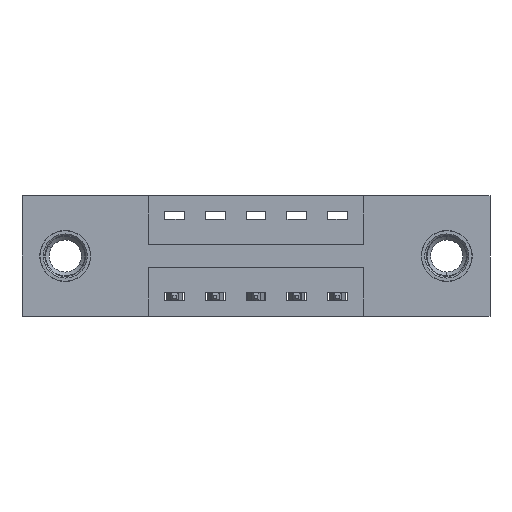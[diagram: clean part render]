
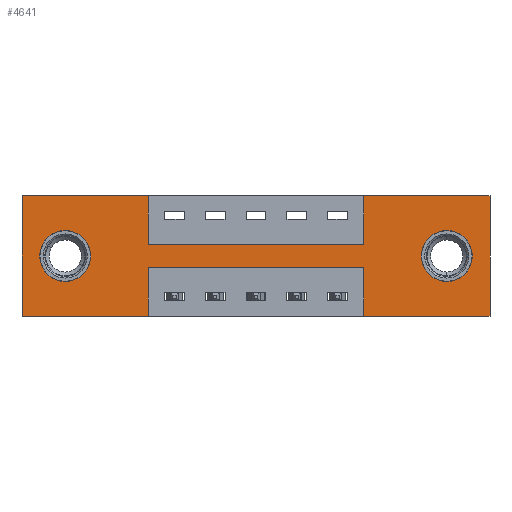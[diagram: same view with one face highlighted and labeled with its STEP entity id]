
A CAD part, front view. The second image highlights one B-rep face of the part: STEP entity #4641.
In plain terms, the highlighted planar face has unit normal (0, -1, 0).
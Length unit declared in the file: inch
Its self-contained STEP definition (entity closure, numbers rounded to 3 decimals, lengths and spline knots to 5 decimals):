
#1 = EDGE_CURVE ( 'NONE', #2073, #1929, #1153, .T. ) ;
#75 = VERTEX_POINT ( 'NONE', #7595 ) ;
#140 = DIRECTION ( 'NONE',  ( 0., 1., 0. ) ) ;
#154 = DIRECTION ( 'NONE',  ( 0., 0., 1. ) ) ;
#171 = CARTESIAN_POINT ( 'NONE',  ( 0.3875, 0., -0.15 ) ) ;
#267 = CARTESIAN_POINT ( 'NONE',  ( 1.3025, 0., -0.185 ) ) ;
#452 = EDGE_CURVE ( 'NONE', #1889, #619, #5421, .T. ) ;
#479 = FACE_OUTER_BOUND ( 'NONE', #673, .T. ) ;
#546 = EDGE_CURVE ( 'NONE', #6700, #4096, #1710, .T. ) ;
#568 = CARTESIAN_POINT ( 'NONE',  ( 0., 0., -0.37 ) ) ;
#619 = VERTEX_POINT ( 'NONE', #7642 ) ;
#673 = EDGE_LOOP ( 'NONE', ( #8582, #4911, #8316, #1388, #771, #6032, #5926, #6555, #3465, #4048, #6415, #8105 ) ) ;
#771 = ORIENTED_EDGE ( 'NONE', *, *, #8049, .F. ) ;
#792 = DIRECTION ( 'NONE',  ( 0., 0., -1. ) ) ;
#867 = CIRCLE ( 'NONE', #6271, 0.078 ) ;
#880 = DIRECTION ( 'NONE',  ( 0., 0., 1. ) ) ;
#926 = EDGE_CURVE ( 'NONE', #4603, #1766, #2413, .T. ) ;
#928 = CARTESIAN_POINT ( 'NONE',  ( 0.1325, 0., -0.185 ) ) ;
#943 = ORIENTED_EDGE ( 'NONE', *, *, #1, .T. ) ;
#967 = VECTOR ( 'NONE', #8298, 39.37008 ) ;
#1014 = EDGE_CURVE ( 'NONE', #8482, #5715, #7037, .T. ) ;
#1153 = CIRCLE ( 'NONE', #4764, 0.078 ) ;
#1210 = CARTESIAN_POINT ( 'NONE',  ( 0.3875, 0., 0. ) ) ;
#1249 = DIRECTION ( 'NONE',  ( 0., 0., 1. ) ) ;
#1314 = CARTESIAN_POINT ( 'NONE',  ( 0.3875, 0., -0.37 ) ) ;
#1388 = ORIENTED_EDGE ( 'NONE', *, *, #452, .F. ) ;
#1443 = VECTOR ( 'NONE', #1249, 39.37008 ) ;
#1526 = VERTEX_POINT ( 'NONE', #2008 ) ;
#1603 = AXIS2_PLACEMENT_3D ( 'NONE', #267, #3846, #1676 ) ;
#1676 = DIRECTION ( 'NONE',  ( 0., 0., -1. ) ) ;
#1710 = LINE ( 'NONE', #7496, #9178 ) ;
#1766 = VERTEX_POINT ( 'NONE', #1314 ) ;
#1817 = DIRECTION ( 'NONE',  ( 0., 0., 1. ) ) ;
#1889 = VERTEX_POINT ( 'NONE', #3568 ) ;
#1929 = VERTEX_POINT ( 'NONE', #2688 ) ;
#2008 = CARTESIAN_POINT ( 'NONE',  ( 0., 0., -0.37 ) ) ;
#2073 = VERTEX_POINT ( 'NONE', #3004 ) ;
#2354 = CARTESIAN_POINT ( 'NONE',  ( 0., 0., 0. ) ) ;
#2413 = LINE ( 'NONE', #4622, #5130 ) ;
#2428 = CARTESIAN_POINT ( 'NONE',  ( 0.1325, 0., -0.185 ) ) ;
#2494 = LINE ( 'NONE', #7371, #6090 ) ;
#2558 = LINE ( 'NONE', #4017, #9057 ) ;
#2571 = CARTESIAN_POINT ( 'NONE',  ( 1.435, 0., 0. ) ) ;
#2614 = DIRECTION ( 'NONE',  ( 1., 0., 0. ) ) ;
#2688 = CARTESIAN_POINT ( 'NONE',  ( 0.1325, 0., -0.263 ) ) ;
#2906 = VECTOR ( 'NONE', #9244, 39.37008 ) ;
#2917 = DIRECTION ( 'NONE',  ( 0., 1., 0. ) ) ;
#2941 = VECTOR ( 'NONE', #6710, 39.37008 ) ;
#2953 = EDGE_CURVE ( 'NONE', #1526, #3997, #8832, .T. ) ;
#3004 = CARTESIAN_POINT ( 'NONE',  ( 0.1325, 0., -0.107 ) ) ;
#3138 = CARTESIAN_POINT ( 'NONE',  ( 0.3875, 0., -0.22 ) ) ;
#3271 = CARTESIAN_POINT ( 'NONE',  ( 1.3025, 0., -0.107 ) ) ;
#3465 = ORIENTED_EDGE ( 'NONE', *, *, #1014, .F. ) ;
#3467 = LINE ( 'NONE', #568, #8217 ) ;
#3568 = CARTESIAN_POINT ( 'NONE',  ( 1.435, 0., -0.37 ) ) ;
#3626 = CARTESIAN_POINT ( 'NONE',  ( 0.3875, 0., 0. ) ) ;
#3767 = LINE ( 'NONE', #2354, #6981 ) ;
#3846 = DIRECTION ( 'NONE',  ( 0., 1., 0. ) ) ;
#3888 = ORIENTED_EDGE ( 'NONE', *, *, #5494, .T. ) ;
#3913 = EDGE_CURVE ( 'NONE', #5715, #5363, #4624, .T. ) ;
#3997 = VERTEX_POINT ( 'NONE', #8749 ) ;
#4017 = CARTESIAN_POINT ( 'NONE',  ( 0.3875, 0., -0.22 ) ) ;
#4048 = ORIENTED_EDGE ( 'NONE', *, *, #9172, .F. ) ;
#4096 = VERTEX_POINT ( 'NONE', #6997 ) ;
#4184 = EDGE_CURVE ( 'NONE', #5244, #75, #7006, .T. ) ;
#4276 = EDGE_LOOP ( 'NONE', ( #943, #7886 ) ) ;
#4366 = CARTESIAN_POINT ( 'NONE',  ( 1.3025, 0., -0.185 ) ) ;
#4512 = CARTESIAN_POINT ( 'NONE',  ( 0., 0., -0.37 ) ) ;
#4603 = VERTEX_POINT ( 'NONE', #3138 ) ;
#4622 = CARTESIAN_POINT ( 'NONE',  ( 0.3875, 0., -0.37 ) ) ;
#4624 = LINE ( 'NONE', #171, #9202 ) ;
#4641 = ADVANCED_FACE ( 'NONE', ( #7649, #8157, #479 ), #5400, .T. ) ;
#4764 = AXIS2_PLACEMENT_3D ( 'NONE', #2428, #140, #880 ) ;
#4772 = CIRCLE ( 'NONE', #1603, 0.078 ) ;
#4829 = CARTESIAN_POINT ( 'NONE',  ( 1.0475, 0., 0. ) ) ;
#4889 = CARTESIAN_POINT ( 'NONE',  ( 1.0475, 0., -0.15 ) ) ;
#4911 = ORIENTED_EDGE ( 'NONE', *, *, #7519, .F. ) ;
#4933 = CARTESIAN_POINT ( 'NONE',  ( 1.0475, 0., -0.22 ) ) ;
#5007 = EDGE_CURVE ( 'NONE', #1766, #1526, #3467, .T. ) ;
#5074 = AXIS2_PLACEMENT_3D ( 'NONE', #7507, #6042, #6729 ) ;
#5130 = VECTOR ( 'NONE', #8275, 39.37008 ) ;
#5193 = DIRECTION ( 'NONE',  ( 1., 0., 0. ) ) ;
#5244 = VERTEX_POINT ( 'NONE', #3271 ) ;
#5315 = VERTEX_POINT ( 'NONE', #4933 ) ;
#5363 = VERTEX_POINT ( 'NONE', #4889 ) ;
#5400 = PLANE ( 'NONE',  #5074 ) ;
#5421 = LINE ( 'NONE', #4512, #8472 ) ;
#5494 = EDGE_CURVE ( 'NONE', #75, #5244, #4772, .T. ) ;
#5602 = EDGE_CURVE ( 'NONE', #5363, #6700, #7029, .T. ) ;
#5715 = VERTEX_POINT ( 'NONE', #8732 ) ;
#5723 = DIRECTION ( 'NONE',  ( -1., 0., 0. ) ) ;
#5782 = EDGE_CURVE ( 'NONE', #1929, #2073, #867, .T. ) ;
#5926 = ORIENTED_EDGE ( 'NONE', *, *, #5602, .F. ) ;
#6032 = ORIENTED_EDGE ( 'NONE', *, *, #546, .F. ) ;
#6042 = DIRECTION ( 'NONE',  ( 0., -1., 0. ) ) ;
#6090 = VECTOR ( 'NONE', #154, 39.37008 ) ;
#6115 = AXIS2_PLACEMENT_3D ( 'NONE', #4366, #2917, #792 ) ;
#6143 = LINE ( 'NONE', #2571, #967 ) ;
#6271 = AXIS2_PLACEMENT_3D ( 'NONE', #928, #8158, #1817 ) ;
#6415 = ORIENTED_EDGE ( 'NONE', *, *, #2953, .F. ) ;
#6555 = ORIENTED_EDGE ( 'NONE', *, *, #3913, .F. ) ;
#6700 = VERTEX_POINT ( 'NONE', #8912 ) ;
#6710 = DIRECTION ( 'NONE',  ( 0., 0., 1. ) ) ;
#6729 = DIRECTION ( 'NONE',  ( 0., 0., -1. ) ) ;
#6758 = ORIENTED_EDGE ( 'NONE', *, *, #4184, .T. ) ;
#6843 = CARTESIAN_POINT ( 'NONE',  ( 0., 0., 0. ) ) ;
#6862 = DIRECTION ( 'NONE',  ( -1., 0., 0. ) ) ;
#6981 = VECTOR ( 'NONE', #5193, 39.37008 ) ;
#6997 = CARTESIAN_POINT ( 'NONE',  ( 1.435, 0., 0. ) ) ;
#7006 = CIRCLE ( 'NONE', #6115, 0.078 ) ;
#7029 = LINE ( 'NONE', #4829, #1443 ) ;
#7037 = LINE ( 'NONE', #1210, #2906 ) ;
#7284 = DIRECTION ( 'NONE',  ( 1., 0., 0. ) ) ;
#7371 = CARTESIAN_POINT ( 'NONE',  ( 1.0475, 0., -0.37 ) ) ;
#7381 = DIRECTION ( 'NONE',  ( -1., 0., 0. ) ) ;
#7496 = CARTESIAN_POINT ( 'NONE',  ( 0., 0., 0. ) ) ;
#7507 = CARTESIAN_POINT ( 'NONE',  ( 0., 0., -0.37 ) ) ;
#7519 = EDGE_CURVE ( 'NONE', #5315, #4603, #2558, .T. ) ;
#7595 = CARTESIAN_POINT ( 'NONE',  ( 1.3025, 0., -0.263 ) ) ;
#7642 = CARTESIAN_POINT ( 'NONE',  ( 1.0475, 0., -0.37 ) ) ;
#7649 = FACE_BOUND ( 'NONE', #9201, .T. ) ;
#7886 = ORIENTED_EDGE ( 'NONE', *, *, #5782, .T. ) ;
#8049 = EDGE_CURVE ( 'NONE', #4096, #1889, #6143, .T. ) ;
#8105 = ORIENTED_EDGE ( 'NONE', *, *, #5007, .F. ) ;
#8157 = FACE_BOUND ( 'NONE', #4276, .T. ) ;
#8158 = DIRECTION ( 'NONE',  ( 0., 1., 0. ) ) ;
#8217 = VECTOR ( 'NONE', #5723, 39.37008 ) ;
#8275 = DIRECTION ( 'NONE',  ( 0., 0., -1. ) ) ;
#8298 = DIRECTION ( 'NONE',  ( 0., 0., -1. ) ) ;
#8316 = ORIENTED_EDGE ( 'NONE', *, *, #9134, .F. ) ;
#8472 = VECTOR ( 'NONE', #7381, 39.37008 ) ;
#8482 = VERTEX_POINT ( 'NONE', #3626 ) ;
#8582 = ORIENTED_EDGE ( 'NONE', *, *, #926, .F. ) ;
#8732 = CARTESIAN_POINT ( 'NONE',  ( 0.3875, 0., -0.15 ) ) ;
#8749 = CARTESIAN_POINT ( 'NONE',  ( 0., 0., 0. ) ) ;
#8832 = LINE ( 'NONE', #6843, #2941 ) ;
#8912 = CARTESIAN_POINT ( 'NONE',  ( 1.0475, 0., 0. ) ) ;
#9057 = VECTOR ( 'NONE', #6862, 39.37008 ) ;
#9134 = EDGE_CURVE ( 'NONE', #619, #5315, #2494, .T. ) ;
#9172 = EDGE_CURVE ( 'NONE', #3997, #8482, #3767, .T. ) ;
#9178 = VECTOR ( 'NONE', #2614, 39.37008 ) ;
#9201 = EDGE_LOOP ( 'NONE', ( #6758, #3888 ) ) ;
#9202 = VECTOR ( 'NONE', #7284, 39.37008 ) ;
#9244 = DIRECTION ( 'NONE',  ( 0., 0., -1. ) ) ;
